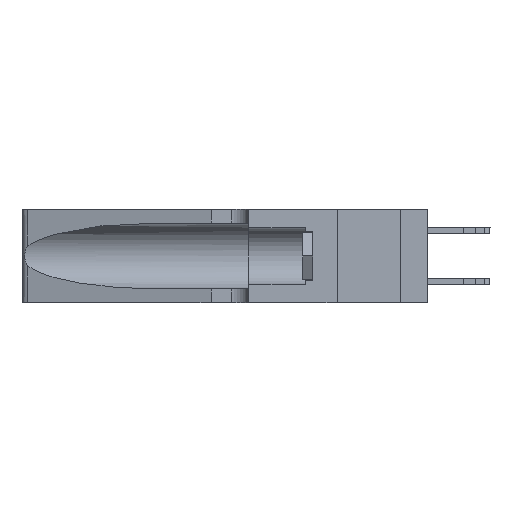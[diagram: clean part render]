
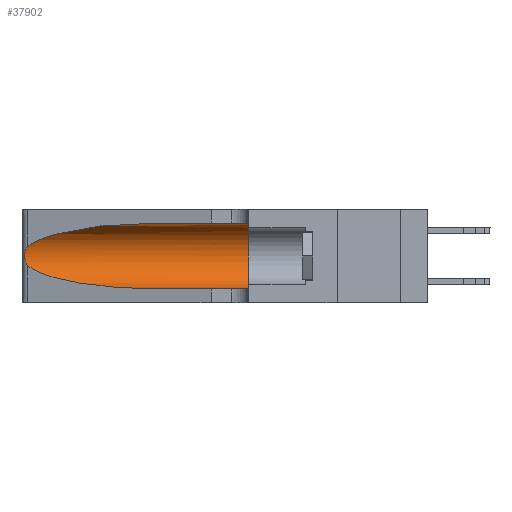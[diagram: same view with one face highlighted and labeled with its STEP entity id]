
A CAD part, left-side view. The second image highlights one B-rep face of the part: STEP entity #37902.
In plain terms, the highlighted cylindrical face has radius 3.308 mm (diameter 6.617 mm), a partial arc.
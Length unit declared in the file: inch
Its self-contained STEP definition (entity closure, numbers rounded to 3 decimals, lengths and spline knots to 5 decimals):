
#272 = CARTESIAN_POINT ( 'NONE',  ( 0.18966, 0.96281, 0.05475 ) ) ;
#606 = ORIENTED_EDGE ( 'NONE', *, *, #26995, .T. ) ;
#772 = ORIENTED_EDGE ( 'NONE', *, *, #3408, .T. ) ;
#944 = CARTESIAN_POINT ( 'NONE',  ( 0.1305, 1.61858, 0.05475 ) ) ;
#2356 = DIRECTION ( 'NONE',  ( 0., 0., 1. ) ) ;
#2743 = LINE ( 'NONE', #4783, #26378 ) ;
#3277 = ORIENTED_EDGE ( 'NONE', *, *, #21529, .F. ) ;
#3408 = EDGE_CURVE ( 'NONE', #15639, #4319, #37618, .T. ) ;
#3583 = EDGE_CURVE ( 'NONE', #21689, #15639, #7635, .T. ) ;
#3712 = VERTEX_POINT ( 'NONE', #19220 ) ;
#4319 = VERTEX_POINT ( 'NONE', #10599 ) ;
#4783 = CARTESIAN_POINT ( 'NONE',  ( 0.1305, 1.61858, 0.31525 ) ) ;
#4876 = CARTESIAN_POINT ( 'NONE',  ( 0.25787, 1.23484, 0.2124 ) ) ;
#6593 = CARTESIAN_POINT ( 'NONE',  ( 0.1305, 0.72297, 0.05475 ) ) ;
#7635 =( BOUNDED_CURVE ( )  B_SPLINE_CURVE ( 3, ( #17416, #11098, #14062, #28871 ),
 .UNSPECIFIED., .F., .F. ) 
 B_SPLINE_CURVE_WITH_KNOTS ( ( 4, 4 ),
 ( 1.5708, 2.84003 ),
 .UNSPECIFIED. ) 
 CURVE ( )  GEOMETRIC_REPRESENTATION_ITEM ( )  RATIONAL_B_SPLINE_CURVE ( ( 1., 0.87, 0.87, 1. ) ) 
 REPRESENTATION_ITEM ( '' )  );
#7842 = CARTESIAN_POINT ( 'NONE',  ( 0.26075, 1.23896, 0.19203 ) ) ;
#8327 = CARTESIAN_POINT ( 'NONE',  ( 0.2373, 1.15595, 0.08982 ) ) ;
#10463 = CARTESIAN_POINT ( 'NONE',  ( 0.25854, 1.2359, 0.20912 ) ) ;
#10599 = CARTESIAN_POINT ( 'NONE',  ( 0.25487, 1.22718, 0.14631 ) ) ;
#10980 = CARTESIAN_POINT ( 'NONE',  ( 0.25639, 1.23186, 0.15144 ) ) ;
#11098 = CARTESIAN_POINT ( 'NONE',  ( 0.18966, 0.96281, 0.31525 ) ) ;
#11196 = ORIENTED_EDGE ( 'NONE', *, *, #28518, .F. ) ;
#12355 = EDGE_LOOP ( 'NONE', ( #19969, #772, #606, #17633, #11196, #3277 ) ) ;
#13428 = CARTESIAN_POINT ( 'NONE',  ( 0.25555, 1.22993, 0.14849 ) ) ;
#13553 = CARTESIAN_POINT ( 'NONE',  ( 0.26018, 1.23835, 0.19895 ) ) ;
#13801 = CARTESIAN_POINT ( 'NONE',  ( 0.25789, 1.23486, 0.15765 ) ) ;
#14062 = CARTESIAN_POINT ( 'NONE',  ( 0.2373, 1.15595, 0.28018 ) ) ;
#15639 = VERTEX_POINT ( 'NONE', #18883 ) ;
#15824 = CARTESIAN_POINT ( 'NONE',  ( 0.1305, 1.61858, 0.185 ) ) ;
#16101 = CIRCLE ( 'NONE', #18252, 0.13025 ) ;
#16761 = CARTESIAN_POINT ( 'NONE',  ( 0.25487, 1.22718, 0.14631 ) ) ;
#16801 = CARTESIAN_POINT ( 'NONE',  ( 0.1305, 0.35, 0.185 ) ) ;
#17416 = CARTESIAN_POINT ( 'NONE',  ( 0.1305, 0.72297, 0.31525 ) ) ;
#17633 = ORIENTED_EDGE ( 'NONE', *, *, #19434, .T. ) ;
#17820 = VECTOR ( 'NONE', #36272, 39.37008 ) ;
#18252 = AXIS2_PLACEMENT_3D ( 'NONE', #16801, #37625, #2356 ) ;
#18744 = FACE_OUTER_BOUND ( 'NONE', #12355, .T. ) ;
#18817 = CARTESIAN_POINT ( 'NONE',  ( 0.1305, 0.35, 0.31525 ) ) ;
#18883 = CARTESIAN_POINT ( 'NONE',  ( 0.25487, 1.22718, 0.22369 ) ) ;
#19220 = CARTESIAN_POINT ( 'NONE',  ( 0.1305, 0.35, 0.05475 ) ) ;
#19434 = EDGE_CURVE ( 'NONE', #31352, #3712, #21545, .T. ) ;
#19634 = CARTESIAN_POINT ( 'NONE',  ( 0.25487, 1.22718, 0.22369 ) ) ;
#19969 = ORIENTED_EDGE ( 'NONE', *, *, #3583, .T. ) ;
#21015 = CARTESIAN_POINT ( 'NONE',  ( 0.1305, 0.72297, 0.05475 ) ) ;
#21529 = EDGE_CURVE ( 'NONE', #21689, #34564, #2743, .T. ) ;
#21545 = LINE ( 'NONE', #944, #17820 ) ;
#21689 = VERTEX_POINT ( 'NONE', #34606 ) ;
#25496 = CARTESIAN_POINT ( 'NONE',  ( 0.26075, 1.23896, 0.178 ) ) ;
#26378 = VECTOR ( 'NONE', #36846, 39.37008 ) ;
#26995 = EDGE_CURVE ( 'NONE', #4319, #31352, #36422, .T. ) ;
#27674 = DIRECTION ( 'NONE',  ( 0., 0., -1. ) ) ;
#28518 = EDGE_CURVE ( 'NONE', #34564, #3712, #16101, .T. ) ;
#28610 = CARTESIAN_POINT ( 'NONE',  ( 0.26017, 1.23833, 0.17102 ) ) ;
#28732 = CARTESIAN_POINT ( 'NONE',  ( 0.25555, 1.22994, 0.2215 ) ) ;
#28871 = CARTESIAN_POINT ( 'NONE',  ( 0.25487, 1.22718, 0.22369 ) ) ;
#28975 = CARTESIAN_POINT ( 'NONE',  ( 0.25487, 1.22718, 0.14631 ) ) ;
#31236 = CARTESIAN_POINT ( 'NONE',  ( 0.25639, 1.23184, 0.21858 ) ) ;
#31352 = VERTEX_POINT ( 'NONE', #6593 ) ;
#34564 = VERTEX_POINT ( 'NONE', #18817 ) ;
#34606 = CARTESIAN_POINT ( 'NONE',  ( 0.1305, 0.72297, 0.31525 ) ) ;
#36272 = DIRECTION ( 'NONE',  ( 0., -1., 0. ) ) ;
#36422 =( BOUNDED_CURVE ( )  B_SPLINE_CURVE ( 3, ( #28975, #8327, #272, #21015 ),
 .UNSPECIFIED., .F., .F. ) 
 B_SPLINE_CURVE_WITH_KNOTS ( ( 4, 4 ),
 ( 3.44316, 4.71239 ),
 .UNSPECIFIED. ) 
 CURVE ( )  GEOMETRIC_REPRESENTATION_ITEM ( )  RATIONAL_B_SPLINE_CURVE ( ( 1., 0.87, 0.87, 1. ) ) 
 REPRESENTATION_ITEM ( '' )  );
#36635 = DIRECTION ( 'NONE',  ( 0., -1., 0. ) ) ;
#36846 = DIRECTION ( 'NONE',  ( 0., -1., 0. ) ) ;
#36927 = CYLINDRICAL_SURFACE ( 'NONE', #37727, 0.13025 ) ;
#37585 = CARTESIAN_POINT ( 'NONE',  ( 0.25856, 1.23593, 0.16098 ) ) ;
#37618 = B_SPLINE_CURVE_WITH_KNOTS ( 'NONE', 3,
 ( #19634, #28732, #31236, #4876, #10463, #13553, #7842, #25496, #28610, #37585, #13801, #10980, #13428, #16761 ),
 .UNSPECIFIED., .F., .F.,
 ( 4, 2, 2, 2, 2, 2, 4 ),
 ( 0., 0.00027, 0.00053, 0.00107, 0.0016, 0.00187, 0.00214 ),
 .UNSPECIFIED. ) ;
#37625 = DIRECTION ( 'NONE',  ( 0., 1., 0. ) ) ;
#37727 = AXIS2_PLACEMENT_3D ( 'NONE', #15824, #36635, #27674 ) ;
#37902 = ADVANCED_FACE ( 'NONE', ( #18744 ), #36927, .F. ) ;
